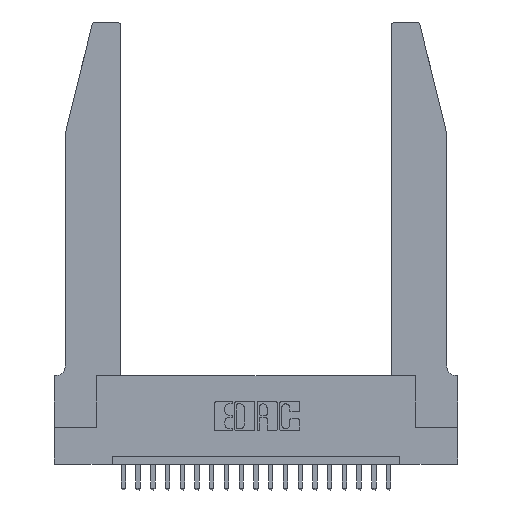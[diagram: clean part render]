
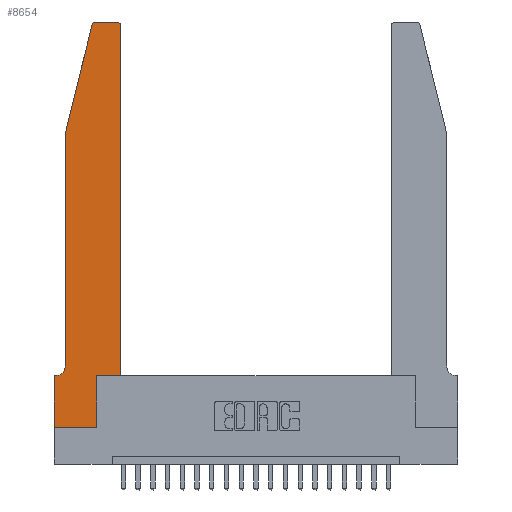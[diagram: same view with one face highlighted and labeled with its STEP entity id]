
A CAD part, top view. The second image highlights one B-rep face of the part: STEP entity #8654.
In plain terms, the highlighted planar face has unit normal (0, 0, 1).
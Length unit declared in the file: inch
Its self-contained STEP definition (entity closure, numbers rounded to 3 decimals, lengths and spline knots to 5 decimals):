
#168 = CARTESIAN_POINT ( 'NONE',  ( 0.25487, 2.72718, 0.37 ) ) ;
#210 = DIRECTION ( 'NONE',  ( -1., 0., 0. ) ) ;
#514 = CARTESIAN_POINT ( 'NONE',  ( 0., 0., 0.37 ) ) ;
#626 = CARTESIAN_POINT ( 'NONE',  ( 0.2865, 0.35, 0.37 ) ) ;
#666 = DIRECTION ( 'NONE',  ( 0., 0., 1. ) ) ;
#710 = DIRECTION ( 'NONE',  ( 0., 0., 1. ) ) ;
#1607 = CARTESIAN_POINT ( 'NONE',  ( 0.0055, 0.42, 0.37 ) ) ;
#2180 = VERTEX_POINT ( 'NONE', #15166 ) ;
#2894 = ORIENTED_EDGE ( 'NONE', *, *, #14144, .T. ) ;
#3107 = VECTOR ( 'NONE', #13245, 39.37008 ) ;
#3348 = ORIENTED_EDGE ( 'NONE', *, *, #11609, .T. ) ;
#3386 = ORIENTED_EDGE ( 'NONE', *, *, #17843, .T. ) ;
#3518 = VERTEX_POINT ( 'NONE', #5767 ) ;
#3552 = CARTESIAN_POINT ( 'NONE',  ( 0.284, 2.75, 0.37 ) ) ;
#3831 = LINE ( 'NONE', #21637, #10530 ) ;
#3875 = CARTESIAN_POINT ( 'NONE',  ( 0.2605, 2.75, 0.37 ) ) ;
#3957 = VERTEX_POINT ( 'NONE', #8192 ) ;
#4143 = LINE ( 'NONE', #8311, #9457 ) ;
#4268 = VECTOR ( 'NONE', #22013, 39.37008 ) ;
#4935 = AXIS2_PLACEMENT_3D ( 'NONE', #1607, #20535, #13701 ) ;
#5138 = EDGE_CURVE ( 'NONE', #21874, #6806, #17684, .T. ) ;
#5206 = CIRCLE ( 'NONE', #10683, 0.03 ) ;
#5685 = EDGE_CURVE ( 'NONE', #6806, #3957, #7182, .T. ) ;
#5704 = CARTESIAN_POINT ( 'NONE',  ( 0.4505, 0.35, 0.37 ) ) ;
#5734 = CARTESIAN_POINT ( 'NONE',  ( 0., 0.35, 0.37 ) ) ;
#5767 = CARTESIAN_POINT ( 'NONE',  ( 0.0755, 0.42, 0.37 ) ) ;
#6213 = CARTESIAN_POINT ( 'NONE',  ( 0., 0., 0.37 ) ) ;
#6259 = DIRECTION ( 'NONE',  ( -1., 0., 0. ) ) ;
#6729 = AXIS2_PLACEMENT_3D ( 'NONE', #5734, #14340, #19156 ) ;
#6806 = VERTEX_POINT ( 'NONE', #13309 ) ;
#6821 = DIRECTION ( 'NONE',  ( -0.239, -0.971, 0. ) ) ;
#7080 = DIRECTION ( 'NONE',  ( 0., -1., 0. ) ) ;
#7182 = CIRCLE ( 'NONE', #18216, 0.03 ) ;
#7211 = EDGE_CURVE ( 'NONE', #11734, #12370, #8444, .T. ) ;
#7378 = ORIENTED_EDGE ( 'NONE', *, *, #8920, .T. ) ;
#8192 = CARTESIAN_POINT ( 'NONE',  ( 0.4205, 2.75, 0.37 ) ) ;
#8311 = CARTESIAN_POINT ( 'NONE',  ( 0.0755, 2., 0.37 ) ) ;
#8444 = LINE ( 'NONE', #19959, #21648 ) ;
#8507 = ORIENTED_EDGE ( 'NONE', *, *, #5138, .T. ) ;
#8654 = ADVANCED_FACE ( 'NONE', ( #11641 ), #12559, .T. ) ;
#8920 = EDGE_CURVE ( 'NONE', #17460, #9069, #4143, .T. ) ;
#9069 = VERTEX_POINT ( 'NONE', #20764 ) ;
#9392 = EDGE_CURVE ( 'NONE', #22223, #2180, #13652, .T. ) ;
#9457 = VECTOR ( 'NONE', #6821, 39.37008 ) ;
#9646 = DIRECTION ( 'NONE',  ( 1., 0., 0. ) ) ;
#10530 = VECTOR ( 'NONE', #6259, 39.37008 ) ;
#10683 = AXIS2_PLACEMENT_3D ( 'NONE', #13328, #666, #21482 ) ;
#11002 = CARTESIAN_POINT ( 'NONE',  ( 0.4205, 2.72, 0.37 ) ) ;
#11382 = EDGE_CURVE ( 'NONE', #2180, #11734, #15688, .T. ) ;
#11609 = EDGE_CURVE ( 'NONE', #3957, #17473, #19451, .T. ) ;
#11641 = FACE_OUTER_BOUND ( 'NONE', #14709, .T. ) ;
#11708 = ORIENTED_EDGE ( 'NONE', *, *, #20784, .T. ) ;
#11734 = VERTEX_POINT ( 'NONE', #12697 ) ;
#11941 = VECTOR ( 'NONE', #210, 39.37008 ) ;
#12044 = LINE ( 'NONE', #20147, #4268 ) ;
#12370 = VERTEX_POINT ( 'NONE', #626 ) ;
#12559 = PLANE ( 'NONE',  #6729 ) ;
#12673 = CIRCLE ( 'NONE', #4935, 0.07 ) ;
#12697 = CARTESIAN_POINT ( 'NONE',  ( 0.2865, 0., 0.37 ) ) ;
#12950 = ORIENTED_EDGE ( 'NONE', *, *, #5685, .T. ) ;
#13245 = DIRECTION ( 'NONE',  ( 1., 0., 0. ) ) ;
#13309 = CARTESIAN_POINT ( 'NONE',  ( 0.4505, 2.72, 0.37 ) ) ;
#13328 = CARTESIAN_POINT ( 'NONE',  ( 0.284, 2.72, 0.37 ) ) ;
#13383 = EDGE_CURVE ( 'NONE', #3518, #19678, #12673, .T. ) ;
#13652 = LINE ( 'NONE', #514, #13889 ) ;
#13701 = DIRECTION ( 'NONE',  ( -1., 0., 0. ) ) ;
#13889 = VECTOR ( 'NONE', #7080, 39.37008 ) ;
#14144 = EDGE_CURVE ( 'NONE', #12370, #21874, #15615, .T. ) ;
#14340 = DIRECTION ( 'NONE',  ( 0., 0., 1. ) ) ;
#14459 = DIRECTION ( 'NONE',  ( 1., 0., 0. ) ) ;
#14492 = CARTESIAN_POINT ( 'NONE',  ( 0.4505, 0.35, 0.37 ) ) ;
#14709 = EDGE_LOOP ( 'NONE', ( #3348, #3386, #7378, #11708, #16339, #15348, #21759, #17578, #16504, #2894, #8507, #12950 ) ) ;
#14726 = VECTOR ( 'NONE', #17824, 39.37008 ) ;
#15166 = CARTESIAN_POINT ( 'NONE',  ( 0., 0., 0.37 ) ) ;
#15348 = ORIENTED_EDGE ( 'NONE', *, *, #17906, .T. ) ;
#15615 = LINE ( 'NONE', #5704, #18565 ) ;
#15688 = LINE ( 'NONE', #6213, #3107 ) ;
#15875 = CARTESIAN_POINT ( 'NONE',  ( 0.4505, 0.35, 0.37 ) ) ;
#16339 = ORIENTED_EDGE ( 'NONE', *, *, #13383, .T. ) ;
#16504 = ORIENTED_EDGE ( 'NONE', *, *, #7211, .T. ) ;
#16744 = DIRECTION ( 'NONE',  ( 0., 1., 0. ) ) ;
#17460 = VERTEX_POINT ( 'NONE', #168 ) ;
#17473 = VERTEX_POINT ( 'NONE', #3552 ) ;
#17578 = ORIENTED_EDGE ( 'NONE', *, *, #11382, .T. ) ;
#17684 = LINE ( 'NONE', #14492, #14726 ) ;
#17824 = DIRECTION ( 'NONE',  ( 0., 1., 0. ) ) ;
#17843 = EDGE_CURVE ( 'NONE', #17473, #17460, #5206, .T. ) ;
#17906 = EDGE_CURVE ( 'NONE', #19678, #22223, #3831, .T. ) ;
#18216 = AXIS2_PLACEMENT_3D ( 'NONE', #11002, #710, #14459 ) ;
#18563 = CARTESIAN_POINT ( 'NONE',  ( 0., 0.35, 0.37 ) ) ;
#18565 = VECTOR ( 'NONE', #9646, 39.37008 ) ;
#18934 = CARTESIAN_POINT ( 'NONE',  ( 0.0055, 0.35, 0.37 ) ) ;
#19156 = DIRECTION ( 'NONE',  ( 1., 0., 0. ) ) ;
#19451 = LINE ( 'NONE', #3875, #11941 ) ;
#19678 = VERTEX_POINT ( 'NONE', #18934 ) ;
#19959 = CARTESIAN_POINT ( 'NONE',  ( 0.2865, 0.35, 0.37 ) ) ;
#20147 = CARTESIAN_POINT ( 'NONE',  ( 0.0755, 2., 0.37 ) ) ;
#20535 = DIRECTION ( 'NONE',  ( 0., 0., -1. ) ) ;
#20764 = CARTESIAN_POINT ( 'NONE',  ( 0.0755, 2., 0.37 ) ) ;
#20784 = EDGE_CURVE ( 'NONE', #9069, #3518, #12044, .T. ) ;
#21482 = DIRECTION ( 'NONE',  ( 1., 0., 0. ) ) ;
#21637 = CARTESIAN_POINT ( 'NONE',  ( 0.0755, 0.35, 0.37 ) ) ;
#21648 = VECTOR ( 'NONE', #16744, 39.37008 ) ;
#21759 = ORIENTED_EDGE ( 'NONE', *, *, #9392, .T. ) ;
#21874 = VERTEX_POINT ( 'NONE', #15875 ) ;
#22013 = DIRECTION ( 'NONE',  ( 0., -1., 0. ) ) ;
#22223 = VERTEX_POINT ( 'NONE', #18563 ) ;
